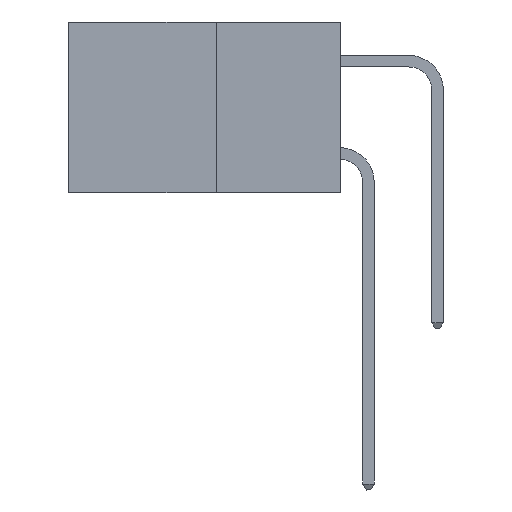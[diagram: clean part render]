
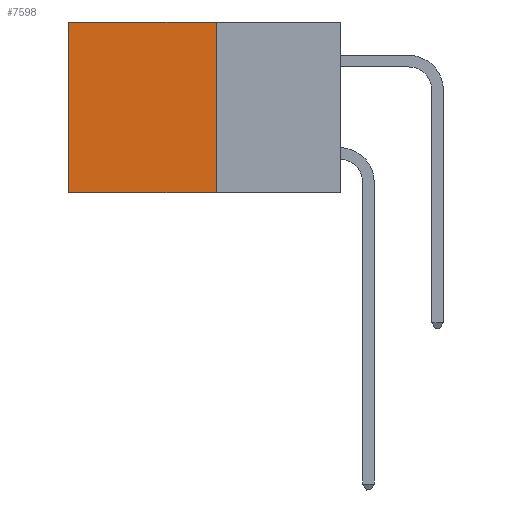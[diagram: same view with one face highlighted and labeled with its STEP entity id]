
A CAD part, left-side view. The second image highlights one B-rep face of the part: STEP entity #7598.
In plain terms, the highlighted planar face has unit normal (-1, 0, 0).
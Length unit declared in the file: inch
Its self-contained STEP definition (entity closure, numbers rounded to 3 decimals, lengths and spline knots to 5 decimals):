
#1351 = CARTESIAN_POINT ( 'NONE',  ( 0.277, 0.27, -0.37 ) ) ;
#2598 = VERTEX_POINT ( 'NONE', #7787 ) ;
#3581 = PLANE ( 'NONE',  #17976 ) ;
#3935 = EDGE_CURVE ( 'NONE', #23898, #11565, #12839, .T. ) ;
#4946 = EDGE_CURVE ( 'NONE', #2598, #11565, #16880, .T. ) ;
#4990 = EDGE_LOOP ( 'NONE', ( #19689, #16786, #4996, #13387 ) ) ;
#4996 = ORIENTED_EDGE ( 'NONE', *, *, #14417, .F. ) ;
#5497 = DIRECTION ( 'NONE',  ( 0., 1., 0. ) ) ;
#6992 = VECTOR ( 'NONE', #18570, 39.37008 ) ;
#7598 = ADVANCED_FACE ( 'NONE', ( #25239 ), #3581, .F. ) ;
#7774 = LINE ( 'NONE', #20740, #12934 ) ;
#7787 = CARTESIAN_POINT ( 'NONE',  ( 0.277, 0.27, -0.37 ) ) ;
#7839 = DIRECTION ( 'NONE',  ( 0., 0., -1. ) ) ;
#7983 = DIRECTION ( 'NONE',  ( 0., 0., -1. ) ) ;
#9715 = CARTESIAN_POINT ( 'NONE',  ( 0.277, 0.59, -0.37 ) ) ;
#11048 = VERTEX_POINT ( 'NONE', #17219 ) ;
#11121 = CARTESIAN_POINT ( 'NONE',  ( 0.277, 0.27, -0.37 ) ) ;
#11565 = VERTEX_POINT ( 'NONE', #9715 ) ;
#12839 = LINE ( 'NONE', #16400, #6992 ) ;
#12934 = VECTOR ( 'NONE', #5497, 39.37008 ) ;
#13332 = DIRECTION ( 'NONE',  ( 0., 1., 0. ) ) ;
#13387 = ORIENTED_EDGE ( 'NONE', *, *, #23285, .T. ) ;
#14417 = EDGE_CURVE ( 'NONE', #11048, #2598, #25331, .T. ) ;
#16400 = CARTESIAN_POINT ( 'NONE',  ( 0.277, 0.59, -0.37 ) ) ;
#16786 = ORIENTED_EDGE ( 'NONE', *, *, #4946, .F. ) ;
#16880 = LINE ( 'NONE', #11121, #23366 ) ;
#17219 = CARTESIAN_POINT ( 'NONE',  ( 0.277, 0.27, 0. ) ) ;
#17976 = AXIS2_PLACEMENT_3D ( 'NONE', #1351, #21036, #7983 ) ;
#18570 = DIRECTION ( 'NONE',  ( 0., 0., -1. ) ) ;
#19689 = ORIENTED_EDGE ( 'NONE', *, *, #3935, .T. ) ;
#20740 = CARTESIAN_POINT ( 'NONE',  ( 0.277, 0.27, 0. ) ) ;
#21036 = DIRECTION ( 'NONE',  ( 1., 0., 0. ) ) ;
#23285 = EDGE_CURVE ( 'NONE', #11048, #23898, #7774, .T. ) ;
#23366 = VECTOR ( 'NONE', #13332, 39.37008 ) ;
#23898 = VERTEX_POINT ( 'NONE', #26895 ) ;
#25239 = FACE_OUTER_BOUND ( 'NONE', #4990, .T. ) ;
#25331 = LINE ( 'NONE', #27528, #26025 ) ;
#26025 = VECTOR ( 'NONE', #7839, 39.37008 ) ;
#26895 = CARTESIAN_POINT ( 'NONE',  ( 0.277, 0.59, 0. ) ) ;
#27528 = CARTESIAN_POINT ( 'NONE',  ( 0.277, 0.27, -0.37 ) ) ;
